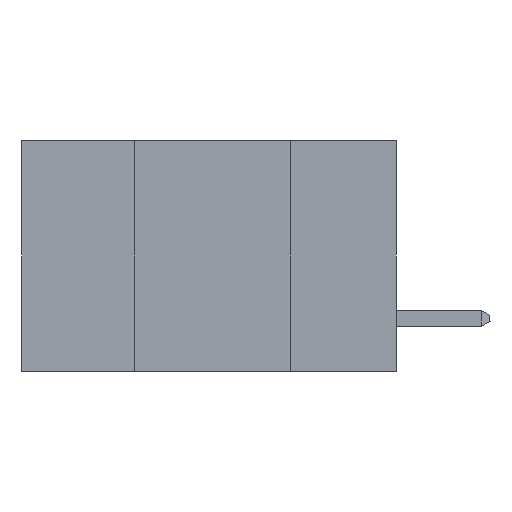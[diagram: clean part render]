
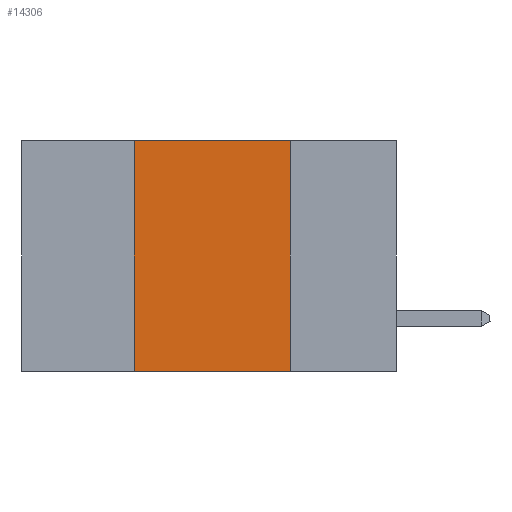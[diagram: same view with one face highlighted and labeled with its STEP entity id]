
A CAD part, left-side view. The second image highlights one B-rep face of the part: STEP entity #14306.
In plain terms, the highlighted planar face has unit normal (-1, 0, 0).
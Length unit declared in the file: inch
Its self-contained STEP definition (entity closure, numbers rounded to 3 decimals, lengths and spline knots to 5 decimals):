
#375 = ORIENTED_EDGE ( 'NONE', *, *, #2309, .F. ) ;
#663 = CARTESIAN_POINT ( 'NONE',  ( 0., 0.42, 0. ) ) ;
#1054 = AXIS2_PLACEMENT_3D ( 'NONE', #2613, #1336, #14759 ) ;
#1104 = VERTEX_POINT ( 'NONE', #16807 ) ;
#1336 = DIRECTION ( 'NONE',  ( 1., 0., 0. ) ) ;
#1793 = EDGE_CURVE ( 'NONE', #6375, #12552, #9824, .T. ) ;
#2252 = VECTOR ( 'NONE', #6266, 39.37008 ) ;
#2309 = EDGE_CURVE ( 'NONE', #17109, #1104, #9378, .T. ) ;
#2613 = CARTESIAN_POINT ( 'NONE',  ( 0., 0.6, 0. ) ) ;
#2705 = VECTOR ( 'NONE', #7941, 39.37008 ) ;
#3494 = VECTOR ( 'NONE', #4660, 39.37008 ) ;
#3612 = EDGE_LOOP ( 'NONE', ( #9251, #375, #11909, #16697 ) ) ;
#3639 = VECTOR ( 'NONE', #12995, 39.37008 ) ;
#4660 = DIRECTION ( 'NONE',  ( 0., -1., 0. ) ) ;
#6060 = FACE_OUTER_BOUND ( 'NONE', #3612, .T. ) ;
#6266 = DIRECTION ( 'NONE',  ( 0., -1., 0. ) ) ;
#6375 = VERTEX_POINT ( 'NONE', #14604 ) ;
#7310 = LINE ( 'NONE', #15884, #2705 ) ;
#7941 = DIRECTION ( 'NONE',  ( 0., 0., 1. ) ) ;
#9251 = ORIENTED_EDGE ( 'NONE', *, *, #11166, .F. ) ;
#9378 = LINE ( 'NONE', #15247, #3494 ) ;
#9824 = LINE ( 'NONE', #11576, #2252 ) ;
#10242 = PLANE ( 'NONE',  #1054 ) ;
#11166 = EDGE_CURVE ( 'NONE', #1104, #12552, #13661, .T. ) ;
#11576 = CARTESIAN_POINT ( 'NONE',  ( 0., 0.6, -0.37 ) ) ;
#11909 = ORIENTED_EDGE ( 'NONE', *, *, #16928, .F. ) ;
#12552 = VERTEX_POINT ( 'NONE', #16755 ) ;
#12939 = CARTESIAN_POINT ( 'NONE',  ( 0., 0.17, 0. ) ) ;
#12995 = DIRECTION ( 'NONE',  ( 0., 0., -1. ) ) ;
#13661 = LINE ( 'NONE', #12939, #3639 ) ;
#14306 = ADVANCED_FACE ( 'NONE', ( #6060 ), #10242, .F. ) ;
#14604 = CARTESIAN_POINT ( 'NONE',  ( 0., 0.42, -0.37 ) ) ;
#14759 = DIRECTION ( 'NONE',  ( 0., 0., -1. ) ) ;
#15247 = CARTESIAN_POINT ( 'NONE',  ( 0., 0.6, 0. ) ) ;
#15884 = CARTESIAN_POINT ( 'NONE',  ( 0., 0.42, 0. ) ) ;
#16697 = ORIENTED_EDGE ( 'NONE', *, *, #1793, .T. ) ;
#16755 = CARTESIAN_POINT ( 'NONE',  ( 0., 0.17, -0.37 ) ) ;
#16807 = CARTESIAN_POINT ( 'NONE',  ( 0., 0.17, 0. ) ) ;
#16928 = EDGE_CURVE ( 'NONE', #6375, #17109, #7310, .T. ) ;
#17109 = VERTEX_POINT ( 'NONE', #663 ) ;
